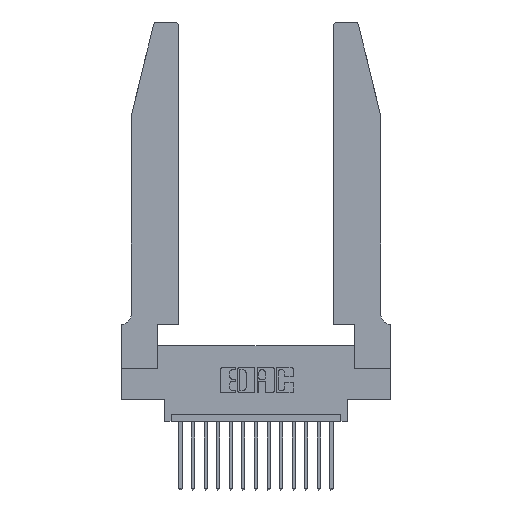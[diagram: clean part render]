
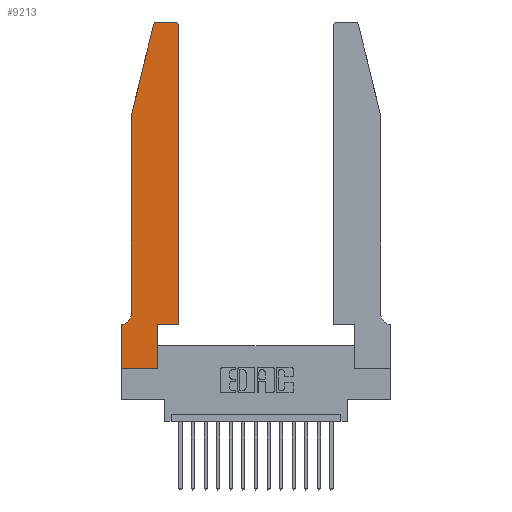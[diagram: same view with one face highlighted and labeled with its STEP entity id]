
A CAD part, top view. The second image highlights one B-rep face of the part: STEP entity #9213.
In plain terms, the highlighted planar face has unit normal (0, 0, 1).
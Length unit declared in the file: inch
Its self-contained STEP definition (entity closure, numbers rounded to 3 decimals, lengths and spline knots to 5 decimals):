
#238 = VERTEX_POINT ( 'NONE', #17138 ) ;
#274 = VERTEX_POINT ( 'NONE', #5971 ) ;
#568 = VERTEX_POINT ( 'NONE', #2905 ) ;
#796 = VECTOR ( 'NONE', #1498, 39.37008 ) ;
#1265 = VERTEX_POINT ( 'NONE', #15728 ) ;
#1318 = DIRECTION ( 'NONE',  ( -1., 0., 0. ) ) ;
#1498 = DIRECTION ( 'NONE',  ( 0., 1., 0. ) ) ;
#1512 = CARTESIAN_POINT ( 'NONE',  ( 0.284, 2.72, 0.37 ) ) ;
#1574 = EDGE_CURVE ( 'NONE', #4050, #4893, #2219, .T. ) ;
#1629 = LINE ( 'NONE', #5923, #8572 ) ;
#1633 = EDGE_LOOP ( 'NONE', ( #16704, #6332, #14136, #13768, #14163, #3178, #11980, #4682, #7160, #1852, #17236, #6860 ) ) ;
#1852 = ORIENTED_EDGE ( 'NONE', *, *, #5058, .T. ) ;
#1859 = LINE ( 'NONE', #14631, #8570 ) ;
#1944 = DIRECTION ( 'NONE',  ( -1., 0., 0. ) ) ;
#2039 = EDGE_CURVE ( 'NONE', #7750, #238, #1629, .T. ) ;
#2219 = LINE ( 'NONE', #3671, #5137 ) ;
#2424 = EDGE_CURVE ( 'NONE', #238, #16674, #8560, .T. ) ;
#2519 = CARTESIAN_POINT ( 'NONE',  ( 0.0755, 2., 0.37 ) ) ;
#2905 = CARTESIAN_POINT ( 'NONE',  ( 0., 0., 0.37 ) ) ;
#3178 = ORIENTED_EDGE ( 'NONE', *, *, #1574, .T. ) ;
#3314 = DIRECTION ( 'NONE',  ( 0., 0., 1. ) ) ;
#3671 = CARTESIAN_POINT ( 'NONE',  ( 0.0755, 0.35, 0.37 ) ) ;
#4048 = LINE ( 'NONE', #8062, #11635 ) ;
#4050 = VERTEX_POINT ( 'NONE', #16319 ) ;
#4562 = VECTOR ( 'NONE', #1944, 39.37008 ) ;
#4682 = ORIENTED_EDGE ( 'NONE', *, *, #12307, .T. ) ;
#4791 = VERTEX_POINT ( 'NONE', #5720 ) ;
#4893 = VERTEX_POINT ( 'NONE', #17357 ) ;
#4933 = EDGE_CURVE ( 'NONE', #1265, #11608, #15462, .T. ) ;
#5058 = EDGE_CURVE ( 'NONE', #274, #7750, #4048, .T. ) ;
#5137 = VECTOR ( 'NONE', #9224, 39.37008 ) ;
#5260 = CARTESIAN_POINT ( 'NONE',  ( 0.4205, 2.75, 0.37 ) ) ;
#5471 = AXIS2_PLACEMENT_3D ( 'NONE', #9835, #3314, #9304 ) ;
#5492 = AXIS2_PLACEMENT_3D ( 'NONE', #1512, #5968, #8815 ) ;
#5720 = CARTESIAN_POINT ( 'NONE',  ( 0.2865, 0., 0.37 ) ) ;
#5923 = CARTESIAN_POINT ( 'NONE',  ( 0.4505, 0.35, 0.37 ) ) ;
#5968 = DIRECTION ( 'NONE',  ( 0., 0., 1. ) ) ;
#5971 = CARTESIAN_POINT ( 'NONE',  ( 0.2865, 0.35, 0.37 ) ) ;
#6057 = DIRECTION ( 'NONE',  ( 0., 1., 0. ) ) ;
#6332 = ORIENTED_EDGE ( 'NONE', *, *, #4933, .T. ) ;
#6860 = ORIENTED_EDGE ( 'NONE', *, *, #2424, .T. ) ;
#7046 = EDGE_CURVE ( 'NONE', #11608, #9033, #18557, .T. ) ;
#7160 = ORIENTED_EDGE ( 'NONE', *, *, #17564, .T. ) ;
#7473 = CARTESIAN_POINT ( 'NONE',  ( 0., 0., 0.37 ) ) ;
#7569 = DIRECTION ( 'NONE',  ( 0., 0., 1. ) ) ;
#7728 = DIRECTION ( 'NONE',  ( 1., 0., 0. ) ) ;
#7750 = VERTEX_POINT ( 'NONE', #11664 ) ;
#8062 = CARTESIAN_POINT ( 'NONE',  ( 0.4505, 0.35, 0.37 ) ) ;
#8133 = AXIS2_PLACEMENT_3D ( 'NONE', #8428, #9878, #1318 ) ;
#8428 = CARTESIAN_POINT ( 'NONE',  ( 0.0055, 0.42, 0.37 ) ) ;
#8508 = CIRCLE ( 'NONE', #8133, 0.07 ) ;
#8560 = CIRCLE ( 'NONE', #10710, 0.03 ) ;
#8570 = VECTOR ( 'NONE', #7728, 39.37008 ) ;
#8572 = VECTOR ( 'NONE', #6057, 39.37008 ) ;
#8735 = CARTESIAN_POINT ( 'NONE',  ( 0.25487, 2.72718, 0.37 ) ) ;
#8815 = DIRECTION ( 'NONE',  ( 1., 0., 0. ) ) ;
#9033 = VERTEX_POINT ( 'NONE', #2519 ) ;
#9213 = ADVANCED_FACE ( 'NONE', ( #15191 ), #16271, .T. ) ;
#9224 = DIRECTION ( 'NONE',  ( -1., 0., 0. ) ) ;
#9304 = DIRECTION ( 'NONE',  ( 1., 0., 0. ) ) ;
#9698 = LINE ( 'NONE', #10513, #4562 ) ;
#9835 = CARTESIAN_POINT ( 'NONE',  ( 0., 0.35, 0.37 ) ) ;
#9878 = DIRECTION ( 'NONE',  ( 0., 0., -1. ) ) ;
#9931 = CARTESIAN_POINT ( 'NONE',  ( 0.2865, 0.35, 0.37 ) ) ;
#9951 = LINE ( 'NONE', #17604, #14432 ) ;
#10156 = VECTOR ( 'NONE', #17526, 39.37008 ) ;
#10513 = CARTESIAN_POINT ( 'NONE',  ( 0.2605, 2.75, 0.37 ) ) ;
#10710 = AXIS2_PLACEMENT_3D ( 'NONE', #16171, #7569, #11685 ) ;
#11200 = DIRECTION ( 'NONE',  ( -0.239, -0.971, 0. ) ) ;
#11413 = CARTESIAN_POINT ( 'NONE',  ( 0.0755, 0.42, 0.37 ) ) ;
#11608 = VERTEX_POINT ( 'NONE', #8735 ) ;
#11635 = VECTOR ( 'NONE', #13807, 39.37008 ) ;
#11664 = CARTESIAN_POINT ( 'NONE',  ( 0.4505, 0.35, 0.37 ) ) ;
#11685 = DIRECTION ( 'NONE',  ( 1., 0., 0. ) ) ;
#11724 = EDGE_CURVE ( 'NONE', #4893, #568, #16694, .T. ) ;
#11775 = VECTOR ( 'NONE', #11200, 39.37008 ) ;
#11980 = ORIENTED_EDGE ( 'NONE', *, *, #11724, .T. ) ;
#12247 = EDGE_CURVE ( 'NONE', #16674, #1265, #9698, .T. ) ;
#12307 = EDGE_CURVE ( 'NONE', #568, #4791, #1859, .T. ) ;
#12529 = VERTEX_POINT ( 'NONE', #11413 ) ;
#13556 = DIRECTION ( 'NONE',  ( 0., -1., 0. ) ) ;
#13768 = ORIENTED_EDGE ( 'NONE', *, *, #17783, .T. ) ;
#13807 = DIRECTION ( 'NONE',  ( 1., 0., 0. ) ) ;
#14136 = ORIENTED_EDGE ( 'NONE', *, *, #7046, .T. ) ;
#14163 = ORIENTED_EDGE ( 'NONE', *, *, #14165, .T. ) ;
#14165 = EDGE_CURVE ( 'NONE', #12529, #4050, #8508, .T. ) ;
#14432 = VECTOR ( 'NONE', #13556, 39.37008 ) ;
#14631 = CARTESIAN_POINT ( 'NONE',  ( 0., 0., 0.37 ) ) ;
#15191 = FACE_OUTER_BOUND ( 'NONE', #1633, .T. ) ;
#15462 = CIRCLE ( 'NONE', #5492, 0.03 ) ;
#15728 = CARTESIAN_POINT ( 'NONE',  ( 0.284, 2.75, 0.37 ) ) ;
#16045 = LINE ( 'NONE', #9931, #796 ) ;
#16171 = CARTESIAN_POINT ( 'NONE',  ( 0.4205, 2.72, 0.37 ) ) ;
#16271 = PLANE ( 'NONE',  #5471 ) ;
#16319 = CARTESIAN_POINT ( 'NONE',  ( 0.0055, 0.35, 0.37 ) ) ;
#16674 = VERTEX_POINT ( 'NONE', #5260 ) ;
#16694 = LINE ( 'NONE', #7473, #10156 ) ;
#16704 = ORIENTED_EDGE ( 'NONE', *, *, #12247, .T. ) ;
#16929 = CARTESIAN_POINT ( 'NONE',  ( 0.0755, 2., 0.37 ) ) ;
#17138 = CARTESIAN_POINT ( 'NONE',  ( 0.4505, 2.72, 0.37 ) ) ;
#17236 = ORIENTED_EDGE ( 'NONE', *, *, #2039, .T. ) ;
#17357 = CARTESIAN_POINT ( 'NONE',  ( 0., 0.35, 0.37 ) ) ;
#17526 = DIRECTION ( 'NONE',  ( 0., -1., 0. ) ) ;
#17564 = EDGE_CURVE ( 'NONE', #4791, #274, #16045, .T. ) ;
#17604 = CARTESIAN_POINT ( 'NONE',  ( 0.0755, 2., 0.37 ) ) ;
#17783 = EDGE_CURVE ( 'NONE', #9033, #12529, #9951, .T. ) ;
#18557 = LINE ( 'NONE', #16929, #11775 ) ;
